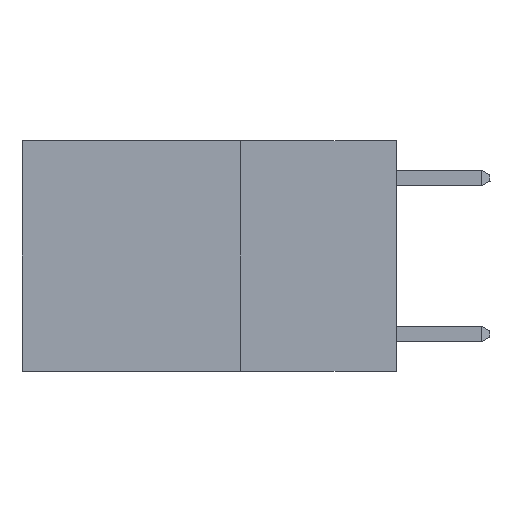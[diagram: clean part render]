
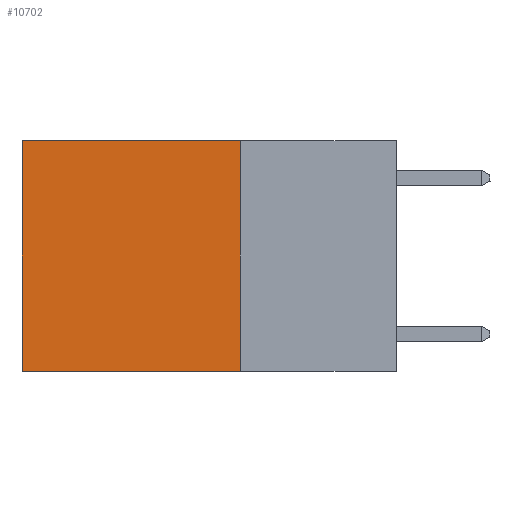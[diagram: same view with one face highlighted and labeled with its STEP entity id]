
A CAD part, left-side view. The second image highlights one B-rep face of the part: STEP entity #10702.
In plain terms, the highlighted planar face has unit normal (-1, 0, 0).
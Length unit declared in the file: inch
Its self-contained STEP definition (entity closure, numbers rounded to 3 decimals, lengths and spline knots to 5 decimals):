
#1922 = VECTOR ( 'NONE', #30188, 39.37008 ) ;
#2168 = CARTESIAN_POINT ( 'NONE',  ( 0.2625, 0.25, 0. ) ) ;
#2631 = DIRECTION ( 'NONE',  ( 0., 1., 0. ) ) ;
#2649 = CARTESIAN_POINT ( 'NONE',  ( 0.2625, 0.6, -0.37 ) ) ;
#3698 = DIRECTION ( 'NONE',  ( 1., 0., 0. ) ) ;
#3796 = EDGE_CURVE ( 'NONE', #6615, #8644, #17411, .T. ) ;
#3807 = DIRECTION ( 'NONE',  ( 0., 0., -1. ) ) ;
#4601 = EDGE_CURVE ( 'NONE', #6615, #21669, #12455, .T. ) ;
#4646 = FACE_OUTER_BOUND ( 'NONE', #30963, .T. ) ;
#4661 = CARTESIAN_POINT ( 'NONE',  ( 0.2625, 0.25, -0.37 ) ) ;
#6009 = VECTOR ( 'NONE', #13517, 39.37008 ) ;
#6615 = VERTEX_POINT ( 'NONE', #2168 ) ;
#8090 = VECTOR ( 'NONE', #2631, 39.37008 ) ;
#8644 = VERTEX_POINT ( 'NONE', #10675 ) ;
#10675 = CARTESIAN_POINT ( 'NONE',  ( 0.2625, 0.25, -0.37 ) ) ;
#10702 = ADVANCED_FACE ( 'NONE', ( #4646 ), #27756, .F. ) ;
#10750 = DIRECTION ( 'NONE',  ( 0., 0., -1. ) ) ;
#10847 = CARTESIAN_POINT ( 'NONE',  ( 0.2625, 0.6, 0. ) ) ;
#12057 = AXIS2_PLACEMENT_3D ( 'NONE', #28093, #3698, #3807 ) ;
#12455 = LINE ( 'NONE', #25423, #6009 ) ;
#13136 = CARTESIAN_POINT ( 'NONE',  ( 0.2625, 0.25, 0. ) ) ;
#13517 = DIRECTION ( 'NONE',  ( 0., 1., 0. ) ) ;
#15180 = ORIENTED_EDGE ( 'NONE', *, *, #28081, .T. ) ;
#15541 = ORIENTED_EDGE ( 'NONE', *, *, #3796, .F. ) ;
#15613 = CARTESIAN_POINT ( 'NONE',  ( 0.2625, 0.6, 0. ) ) ;
#17411 = LINE ( 'NONE', #13136, #1922 ) ;
#18890 = VERTEX_POINT ( 'NONE', #2649 ) ;
#21662 = LINE ( 'NONE', #10847, #29203 ) ;
#21669 = VERTEX_POINT ( 'NONE', #15613 ) ;
#25423 = CARTESIAN_POINT ( 'NONE',  ( 0.2625, 0.25, 0. ) ) ;
#26893 = LINE ( 'NONE', #4661, #8090 ) ;
#27756 = PLANE ( 'NONE',  #12057 ) ;
#28081 = EDGE_CURVE ( 'NONE', #21669, #18890, #21662, .T. ) ;
#28093 = CARTESIAN_POINT ( 'NONE',  ( 0.2625, 0.25, 0. ) ) ;
#28536 = EDGE_CURVE ( 'NONE', #8644, #18890, #26893, .T. ) ;
#29203 = VECTOR ( 'NONE', #10750, 39.37008 ) ;
#29994 = ORIENTED_EDGE ( 'NONE', *, *, #4601, .T. ) ;
#30188 = DIRECTION ( 'NONE',  ( 0., 0., -1. ) ) ;
#30440 = ORIENTED_EDGE ( 'NONE', *, *, #28536, .F. ) ;
#30963 = EDGE_LOOP ( 'NONE', ( #15180, #30440, #15541, #29994 ) ) ;
